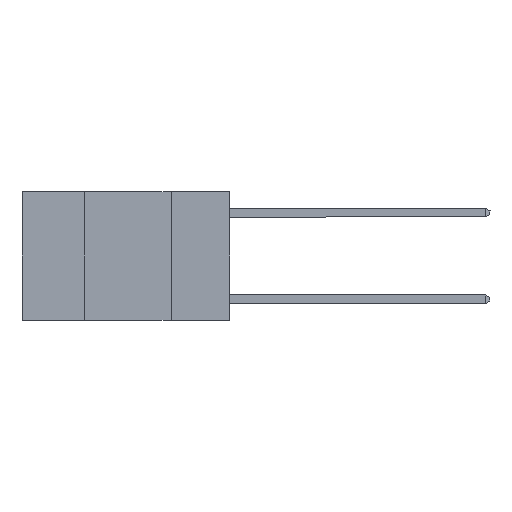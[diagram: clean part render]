
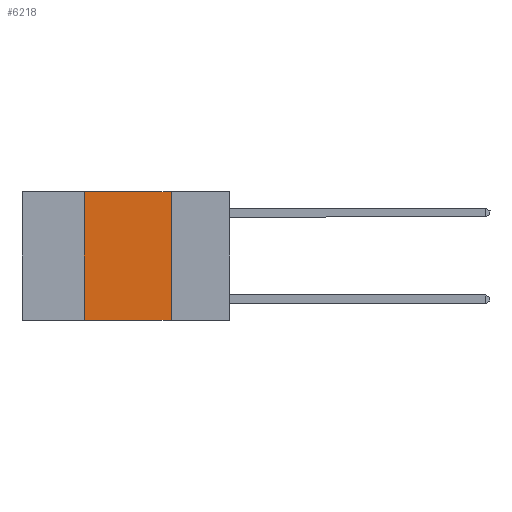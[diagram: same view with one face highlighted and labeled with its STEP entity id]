
A CAD part, left-side view. The second image highlights one B-rep face of the part: STEP entity #6218.
In plain terms, the highlighted planar face has unit normal (-1, 0, 0).
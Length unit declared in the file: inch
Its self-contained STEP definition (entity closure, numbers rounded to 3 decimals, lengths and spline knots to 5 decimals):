
#29 = VERTEX_POINT ( 'NONE', #8442 ) ;
#594 = EDGE_CURVE ( 'NONE', #8763, #29, #5701, .T. ) ;
#642 = ORIENTED_EDGE ( 'NONE', *, *, #5610, .F. ) ;
#817 = EDGE_LOOP ( 'NONE', ( #8689, #642, #1842, #8549 ) ) ;
#933 = FACE_OUTER_BOUND ( 'NONE', #817, .T. ) ;
#1329 = CARTESIAN_POINT ( 'NONE',  ( 0., 0.6, 0. ) ) ;
#1602 = EDGE_CURVE ( 'NONE', #8763, #8847, #2969, .T. ) ;
#1842 = ORIENTED_EDGE ( 'NONE', *, *, #594, .F. ) ;
#2069 = DIRECTION ( 'NONE',  ( 0., 0., -1. ) ) ;
#2328 = AXIS2_PLACEMENT_3D ( 'NONE', #1329, #6505, #2069 ) ;
#2752 = DIRECTION ( 'NONE',  ( 0., -1., 0. ) ) ;
#2770 = VECTOR ( 'NONE', #4897, 39.37008 ) ;
#2969 = LINE ( 'NONE', #8939, #8483 ) ;
#3007 = LINE ( 'NONE', #5670, #2770 ) ;
#3580 = CARTESIAN_POINT ( 'NONE',  ( 0., 0.17, -0.37 ) ) ;
#3762 = VECTOR ( 'NONE', #6451, 39.37008 ) ;
#4159 = CARTESIAN_POINT ( 'NONE',  ( 0., 0.17, 0. ) ) ;
#4201 = VERTEX_POINT ( 'NONE', #4159 ) ;
#4767 = CARTESIAN_POINT ( 'NONE',  ( 0., 0.42, 0. ) ) ;
#4893 = EDGE_CURVE ( 'NONE', #4201, #8847, #3007, .T. ) ;
#4897 = DIRECTION ( 'NONE',  ( 0., 0., -1. ) ) ;
#5610 = EDGE_CURVE ( 'NONE', #29, #4201, #8173, .T. ) ;
#5670 = CARTESIAN_POINT ( 'NONE',  ( 0., 0.17, 0. ) ) ;
#5701 = LINE ( 'NONE', #4767, #3762 ) ;
#5715 = PLANE ( 'NONE',  #2328 ) ;
#6060 = VECTOR ( 'NONE', #2752, 39.37008 ) ;
#6218 = ADVANCED_FACE ( 'NONE', ( #933 ), #5715, .F. ) ;
#6451 = DIRECTION ( 'NONE',  ( 0., 0., 1. ) ) ;
#6461 = CARTESIAN_POINT ( 'NONE',  ( 0., 0.42, -0.37 ) ) ;
#6505 = DIRECTION ( 'NONE',  ( 1., 0., 0. ) ) ;
#7830 = CARTESIAN_POINT ( 'NONE',  ( 0., 0.6, 0. ) ) ;
#8173 = LINE ( 'NONE', #7830, #6060 ) ;
#8442 = CARTESIAN_POINT ( 'NONE',  ( 0., 0.42, 0. ) ) ;
#8483 = VECTOR ( 'NONE', #8723, 39.37008 ) ;
#8549 = ORIENTED_EDGE ( 'NONE', *, *, #1602, .T. ) ;
#8689 = ORIENTED_EDGE ( 'NONE', *, *, #4893, .F. ) ;
#8723 = DIRECTION ( 'NONE',  ( 0., -1., 0. ) ) ;
#8763 = VERTEX_POINT ( 'NONE', #6461 ) ;
#8847 = VERTEX_POINT ( 'NONE', #3580 ) ;
#8939 = CARTESIAN_POINT ( 'NONE',  ( 0., 0.6, -0.37 ) ) ;
